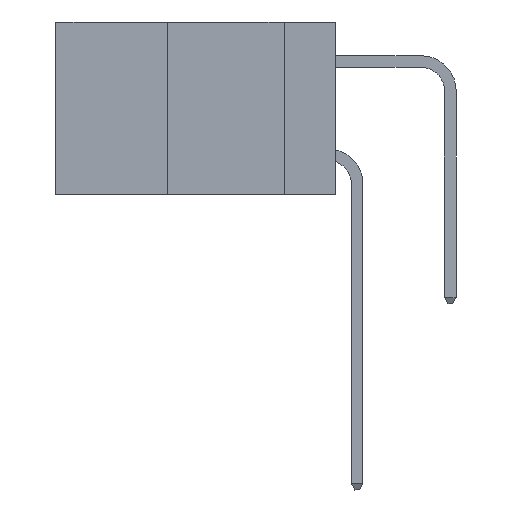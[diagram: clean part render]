
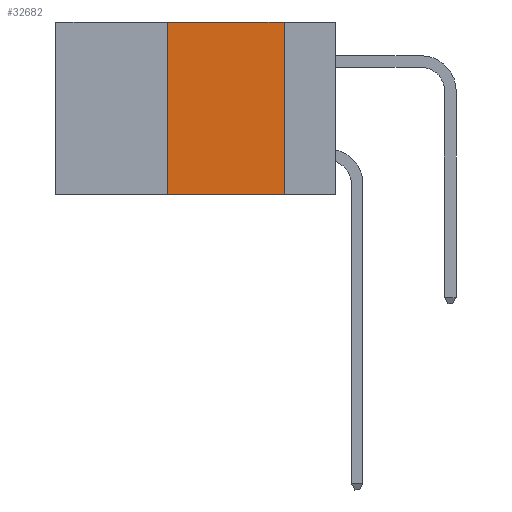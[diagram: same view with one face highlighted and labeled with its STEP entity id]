
A CAD part, left-side view. The second image highlights one B-rep face of the part: STEP entity #32682.
In plain terms, the highlighted planar face has unit normal (-1, 0, 0).
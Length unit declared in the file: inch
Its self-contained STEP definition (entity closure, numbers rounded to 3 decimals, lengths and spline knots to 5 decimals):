
#3823 = DIRECTION ( 'NONE',  ( 0., -1., 0. ) ) ;
#4491 = VERTEX_POINT ( 'NONE', #15420 ) ;
#4971 = DIRECTION ( 'NONE',  ( 1., 0., 0. ) ) ;
#5253 = PLANE ( 'NONE',  #38456 ) ;
#6172 = EDGE_LOOP ( 'NONE', ( #32311, #27383, #7946, #34907 ) ) ;
#7318 = EDGE_CURVE ( 'NONE', #22908, #24336, #10123, .T. ) ;
#7946 = ORIENTED_EDGE ( 'NONE', *, *, #8066, .F. ) ;
#8066 = EDGE_CURVE ( 'NONE', #22908, #4491, #8517, .T. ) ;
#8517 = LINE ( 'NONE', #27474, #9544 ) ;
#8718 = CARTESIAN_POINT ( 'NONE',  ( 0., 0.6, 0. ) ) ;
#8908 = CARTESIAN_POINT ( 'NONE',  ( 0., 0.11, 0. ) ) ;
#9544 = VECTOR ( 'NONE', #34160, 39.37008 ) ;
#10123 = LINE ( 'NONE', #30193, #25308 ) ;
#11806 = DIRECTION ( 'NONE',  ( 0., 0., -1. ) ) ;
#14695 = EDGE_CURVE ( 'NONE', #38198, #24336, #14974, .T. ) ;
#14974 = LINE ( 'NONE', #8908, #18071 ) ;
#15420 = CARTESIAN_POINT ( 'NONE',  ( 0., 0.36, 0. ) ) ;
#15498 = CARTESIAN_POINT ( 'NONE',  ( 0., 0.36, -0.37 ) ) ;
#16125 = VECTOR ( 'NONE', #29118, 39.37008 ) ;
#18071 = VECTOR ( 'NONE', #22363, 39.37008 ) ;
#22363 = DIRECTION ( 'NONE',  ( 0., 0., -1. ) ) ;
#22908 = VERTEX_POINT ( 'NONE', #15498 ) ;
#24336 = VERTEX_POINT ( 'NONE', #41046 ) ;
#25308 = VECTOR ( 'NONE', #3823, 39.37008 ) ;
#27383 = ORIENTED_EDGE ( 'NONE', *, *, #41473, .F. ) ;
#27474 = CARTESIAN_POINT ( 'NONE',  ( 0., 0.36, 0. ) ) ;
#29118 = DIRECTION ( 'NONE',  ( 0., -1., 0. ) ) ;
#29139 = CARTESIAN_POINT ( 'NONE',  ( 0., 0.11, 0. ) ) ;
#29140 = LINE ( 'NONE', #29251, #16125 ) ;
#29251 = CARTESIAN_POINT ( 'NONE',  ( 0., 0.6, 0. ) ) ;
#30193 = CARTESIAN_POINT ( 'NONE',  ( 0., 0.6, -0.37 ) ) ;
#32311 = ORIENTED_EDGE ( 'NONE', *, *, #14695, .F. ) ;
#32682 = ADVANCED_FACE ( 'NONE', ( #37960 ), #5253, .F. ) ;
#34160 = DIRECTION ( 'NONE',  ( 0., 0., 1. ) ) ;
#34907 = ORIENTED_EDGE ( 'NONE', *, *, #7318, .T. ) ;
#37960 = FACE_OUTER_BOUND ( 'NONE', #6172, .T. ) ;
#38198 = VERTEX_POINT ( 'NONE', #29139 ) ;
#38456 = AXIS2_PLACEMENT_3D ( 'NONE', #8718, #4971, #11806 ) ;
#41046 = CARTESIAN_POINT ( 'NONE',  ( 0., 0.11, -0.37 ) ) ;
#41473 = EDGE_CURVE ( 'NONE', #4491, #38198, #29140, .T. ) ;
